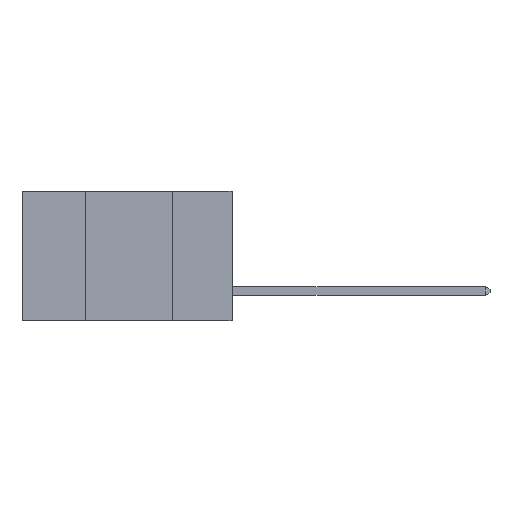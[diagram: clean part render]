
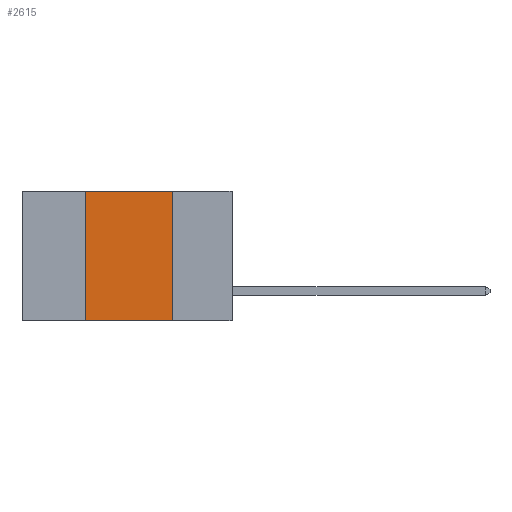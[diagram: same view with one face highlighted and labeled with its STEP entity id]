
A CAD part, left-side view. The second image highlights one B-rep face of the part: STEP entity #2615.
In plain terms, the highlighted planar face has unit normal (-1, 0, 0).
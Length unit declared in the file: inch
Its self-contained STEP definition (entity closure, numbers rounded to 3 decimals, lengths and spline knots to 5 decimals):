
#319 = ORIENTED_EDGE ( 'NONE', *, *, #24893, .F. ) ;
#587 = ORIENTED_EDGE ( 'NONE', *, *, #24775, .T. ) ;
#1188 = VECTOR ( 'NONE', #8742, 39.37008 ) ;
#2615 = ADVANCED_FACE ( 'NONE', ( #23631 ), #27274, .F. ) ;
#3717 = DIRECTION ( 'NONE',  ( 0., 0., 1. ) ) ;
#4012 = DIRECTION ( 'NONE',  ( 0., -1., 0. ) ) ;
#4356 = EDGE_LOOP ( 'NONE', ( #26095, #15230, #319, #587 ) ) ;
#4863 = VERTEX_POINT ( 'NONE', #7944 ) ;
#5495 = CARTESIAN_POINT ( 'NONE',  ( 0., 0.6, -0.37 ) ) ;
#6281 = DIRECTION ( 'NONE',  ( 0., 0., -1. ) ) ;
#6600 = CARTESIAN_POINT ( 'NONE',  ( 0., 0.17, 0. ) ) ;
#7068 = VERTEX_POINT ( 'NONE', #17374 ) ;
#7944 = CARTESIAN_POINT ( 'NONE',  ( 0., 0.17, 0. ) ) ;
#8742 = DIRECTION ( 'NONE',  ( 0., 0., -1. ) ) ;
#8886 = CARTESIAN_POINT ( 'NONE',  ( 0., 0.42, 0. ) ) ;
#9534 = VECTOR ( 'NONE', #18116, 39.37008 ) ;
#9562 = LINE ( 'NONE', #25100, #15823 ) ;
#10035 = CARTESIAN_POINT ( 'NONE',  ( 0., 0.42, 0. ) ) ;
#12559 = CARTESIAN_POINT ( 'NONE',  ( 0., 0.6, 0. ) ) ;
#13290 = CARTESIAN_POINT ( 'NONE',  ( 0., 0.17, -0.37 ) ) ;
#13741 = VERTEX_POINT ( 'NONE', #13290 ) ;
#14233 = EDGE_CURVE ( 'NONE', #4863, #13741, #18051, .T. ) ;
#15230 = ORIENTED_EDGE ( 'NONE', *, *, #24330, .F. ) ;
#15823 = VECTOR ( 'NONE', #4012, 39.37008 ) ;
#16753 = LINE ( 'NONE', #10035, #21103 ) ;
#17374 = CARTESIAN_POINT ( 'NONE',  ( 0., 0.42, -0.37 ) ) ;
#18051 = LINE ( 'NONE', #6600, #1188 ) ;
#18116 = DIRECTION ( 'NONE',  ( 0., -1., 0. ) ) ;
#18738 = LINE ( 'NONE', #5495, #9534 ) ;
#18908 = DIRECTION ( 'NONE',  ( 1., 0., 0. ) ) ;
#20385 = VERTEX_POINT ( 'NONE', #8886 ) ;
#21103 = VECTOR ( 'NONE', #3717, 39.37008 ) ;
#22323 = AXIS2_PLACEMENT_3D ( 'NONE', #12559, #18908, #6281 ) ;
#23631 = FACE_OUTER_BOUND ( 'NONE', #4356, .T. ) ;
#24330 = EDGE_CURVE ( 'NONE', #20385, #4863, #9562, .T. ) ;
#24775 = EDGE_CURVE ( 'NONE', #7068, #13741, #18738, .T. ) ;
#24893 = EDGE_CURVE ( 'NONE', #7068, #20385, #16753, .T. ) ;
#25100 = CARTESIAN_POINT ( 'NONE',  ( 0., 0.6, 0. ) ) ;
#26095 = ORIENTED_EDGE ( 'NONE', *, *, #14233, .F. ) ;
#27274 = PLANE ( 'NONE',  #22323 ) ;
